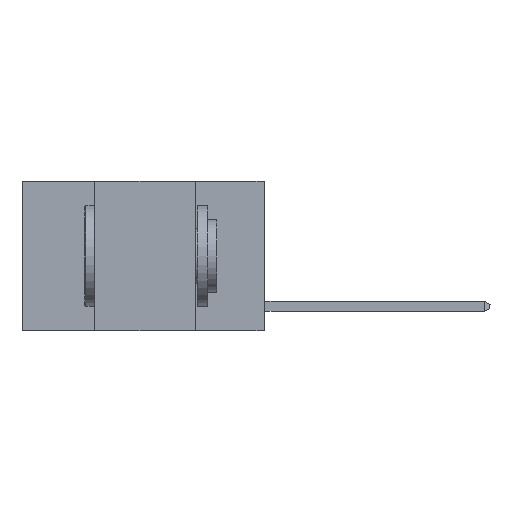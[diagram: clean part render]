
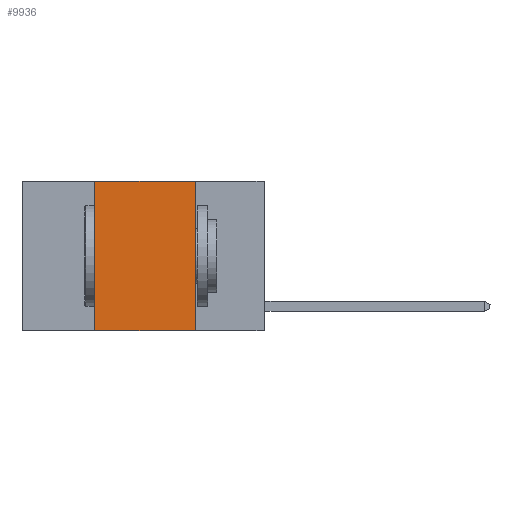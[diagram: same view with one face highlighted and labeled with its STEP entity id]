
A CAD part, left-side view. The second image highlights one B-rep face of the part: STEP entity #9936.
In plain terms, the highlighted planar face has unit normal (-1, 0, 0).
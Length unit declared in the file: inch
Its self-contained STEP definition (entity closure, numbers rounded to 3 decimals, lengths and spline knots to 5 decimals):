
#612 = DIRECTION ( 'NONE',  ( 0., 0., -1. ) ) ;
#1040 = ORIENTED_EDGE ( 'NONE', *, *, #9471, .F. ) ;
#1219 = DIRECTION ( 'NONE',  ( 1., 0., 0. ) ) ;
#1926 = ORIENTED_EDGE ( 'NONE', *, *, #5740, .F. ) ;
#2015 = ORIENTED_EDGE ( 'NONE', *, *, #5737, .T. ) ;
#2508 = LINE ( 'NONE', #6784, #13848 ) ;
#2689 = CARTESIAN_POINT ( 'NONE',  ( 0., 0.6, -0.37 ) ) ;
#2922 = FACE_OUTER_BOUND ( 'NONE', #13255, .T. ) ;
#3803 = VECTOR ( 'NONE', #612, 39.37008 ) ;
#4017 = CARTESIAN_POINT ( 'NONE',  ( 0., 0.17, -0.37 ) ) ;
#4593 = LINE ( 'NONE', #11634, #9902 ) ;
#4658 = AXIS2_PLACEMENT_3D ( 'NONE', #10186, #1219, #5760 ) ;
#4693 = EDGE_CURVE ( 'NONE', #8439, #6574, #2508, .T. ) ;
#4788 = CARTESIAN_POINT ( 'NONE',  ( 0., 0.17, 0. ) ) ;
#4987 = DIRECTION ( 'NONE',  ( 0., 0., 1. ) ) ;
#5737 = EDGE_CURVE ( 'NONE', #6361, #9067, #14194, .T. ) ;
#5740 = EDGE_CURVE ( 'NONE', #6361, #8439, #4593, .T. ) ;
#5760 = DIRECTION ( 'NONE',  ( 0., 0., -1. ) ) ;
#5848 = CARTESIAN_POINT ( 'NONE',  ( 0., 0.42, 0. ) ) ;
#6361 = VERTEX_POINT ( 'NONE', #7797 ) ;
#6521 = DIRECTION ( 'NONE',  ( 0., -1., 0. ) ) ;
#6574 = VERTEX_POINT ( 'NONE', #4788 ) ;
#6784 = CARTESIAN_POINT ( 'NONE',  ( 0., 0.6, 0. ) ) ;
#7797 = CARTESIAN_POINT ( 'NONE',  ( 0., 0.42, -0.37 ) ) ;
#7899 = LINE ( 'NONE', #11618, #3803 ) ;
#8332 = VECTOR ( 'NONE', #13650, 39.37008 ) ;
#8439 = VERTEX_POINT ( 'NONE', #5848 ) ;
#9067 = VERTEX_POINT ( 'NONE', #4017 ) ;
#9471 = EDGE_CURVE ( 'NONE', #6574, #9067, #7899, .T. ) ;
#9902 = VECTOR ( 'NONE', #4987, 39.37008 ) ;
#9936 = ADVANCED_FACE ( 'NONE', ( #2922 ), #12291, .F. ) ;
#10186 = CARTESIAN_POINT ( 'NONE',  ( 0., 0.6, 0. ) ) ;
#10667 = ORIENTED_EDGE ( 'NONE', *, *, #4693, .F. ) ;
#11618 = CARTESIAN_POINT ( 'NONE',  ( 0., 0.17, 0. ) ) ;
#11634 = CARTESIAN_POINT ( 'NONE',  ( 0., 0.42, 0. ) ) ;
#12291 = PLANE ( 'NONE',  #4658 ) ;
#13255 = EDGE_LOOP ( 'NONE', ( #1040, #10667, #1926, #2015 ) ) ;
#13650 = DIRECTION ( 'NONE',  ( 0., -1., 0. ) ) ;
#13848 = VECTOR ( 'NONE', #6521, 39.37008 ) ;
#14194 = LINE ( 'NONE', #2689, #8332 ) ;
